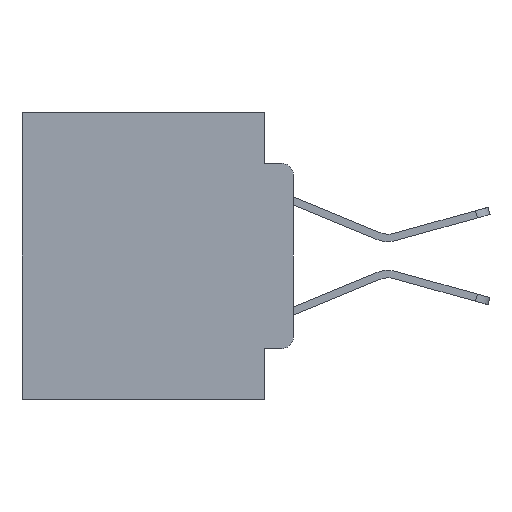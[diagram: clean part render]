
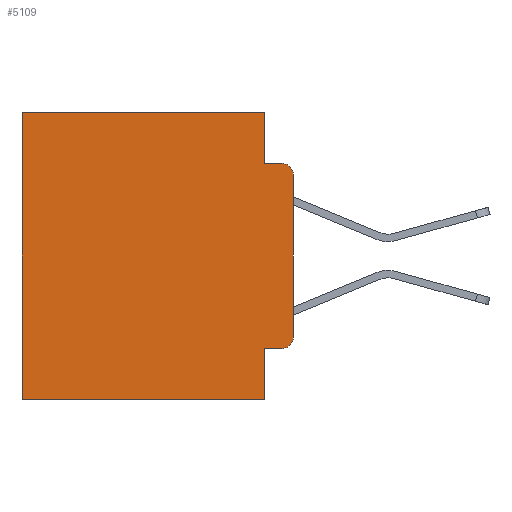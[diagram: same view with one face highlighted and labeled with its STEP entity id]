
A CAD part, left-side view. The second image highlights one B-rep face of the part: STEP entity #5109.
In plain terms, the highlighted planar face has unit normal (-1, 0, 0).
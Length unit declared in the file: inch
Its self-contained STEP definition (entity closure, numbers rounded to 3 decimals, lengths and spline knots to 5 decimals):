
#487 = CARTESIAN_POINT ( 'NONE',  ( 0.298, 0., -0.3915 ) ) ;
#726 = CARTESIAN_POINT ( 'NONE',  ( 0.298, 0.051, -0.4115 ) ) ;
#761 = CARTESIAN_POINT ( 'NONE',  ( 0.298, 0.051, 0. ) ) ;
#1875 = FACE_OUTER_BOUND ( 'NONE', #4667, .T. ) ;
#1947 = CARTESIAN_POINT ( 'NONE',  ( 0.298, 0., 0. ) ) ;
#2018 = PLANE ( 'NONE',  #2571 ) ;
#2416 = VERTEX_POINT ( 'NONE', #8636 ) ;
#2571 = AXIS2_PLACEMENT_3D ( 'NONE', #26349, #21412, #23590 ) ;
#2911 = CARTESIAN_POINT ( 'NONE',  ( 0.298, 0., -0.5 ) ) ;
#3122 = CARTESIAN_POINT ( 'NONE',  ( 0.298, 0.473, 0. ) ) ;
#3281 = DIRECTION ( 'NONE',  ( -1., 0., 0. ) ) ;
#4502 = CARTESIAN_POINT ( 'NONE',  ( 0.298, 0.051, -0.4115 ) ) ;
#4667 = EDGE_LOOP ( 'NONE', ( #11362, #19596, #18901, #5323, #28668, #21080, #15836, #21232, #6042, #21075 ) ) ;
#4672 = EDGE_CURVE ( 'NONE', #19075, #25026, #17510, .T. ) ;
#4812 = VERTEX_POINT ( 'NONE', #4502 ) ;
#4886 = EDGE_CURVE ( 'NONE', #25026, #22188, #6840, .T. ) ;
#4969 = EDGE_CURVE ( 'NONE', #4812, #14832, #7862, .T. ) ;
#5070 = LINE ( 'NONE', #6994, #20782 ) ;
#5094 = CARTESIAN_POINT ( 'NONE',  ( 0.298, 0.02, -0.1085 ) ) ;
#5109 = ADVANCED_FACE ( 'NONE', ( #1875 ), #2018, .F. ) ;
#5323 = ORIENTED_EDGE ( 'NONE', *, *, #4672, .F. ) ;
#5459 = DIRECTION ( 'NONE',  ( 0., 0., -1. ) ) ;
#6042 = ORIENTED_EDGE ( 'NONE', *, *, #4969, .T. ) ;
#6248 = EDGE_CURVE ( 'NONE', #2416, #8622, #24770, .T. ) ;
#6403 = DIRECTION ( 'NONE',  ( 0., 0., -1. ) ) ;
#6766 = CIRCLE ( 'NONE', #7236, 0.02 ) ;
#6840 = LINE ( 'NONE', #15747, #26697 ) ;
#6994 = CARTESIAN_POINT ( 'NONE',  ( 0.298, 0., 0. ) ) ;
#7236 = AXIS2_PLACEMENT_3D ( 'NONE', #17008, #3281, #5459 ) ;
#7862 = LINE ( 'NONE', #726, #8117 ) ;
#8117 = VECTOR ( 'NONE', #18513, 39.37008 ) ;
#8444 = VERTEX_POINT ( 'NONE', #3122 ) ;
#8481 = LINE ( 'NONE', #25953, #27718 ) ;
#8622 = VERTEX_POINT ( 'NONE', #25721 ) ;
#8636 = CARTESIAN_POINT ( 'NONE',  ( 0.298, 0.051, -0.5 ) ) ;
#9099 = VECTOR ( 'NONE', #18489, 39.37008 ) ;
#9623 = LINE ( 'NONE', #11943, #9099 ) ;
#10792 = EDGE_CURVE ( 'NONE', #17193, #22188, #22730, .T. ) ;
#11362 = ORIENTED_EDGE ( 'NONE', *, *, #19406, .F. ) ;
#11943 = CARTESIAN_POINT ( 'NONE',  ( 0.298, 0.473, 0. ) ) ;
#13331 = EDGE_CURVE ( 'NONE', #19075, #8444, #19744, .T. ) ;
#13599 = DIRECTION ( 'NONE',  ( 0., 0., -1. ) ) ;
#14070 = CARTESIAN_POINT ( 'NONE',  ( 0.298, 0.02, -0.4115 ) ) ;
#14832 = VERTEX_POINT ( 'NONE', #14070 ) ;
#15746 = DIRECTION ( 'NONE',  ( 0., 0., -1. ) ) ;
#15747 = CARTESIAN_POINT ( 'NONE',  ( 0.298, 0.051, -0.0885 ) ) ;
#15836 = ORIENTED_EDGE ( 'NONE', *, *, #6248, .F. ) ;
#15892 = EDGE_CURVE ( 'NONE', #8444, #8622, #9623, .T. ) ;
#17008 = CARTESIAN_POINT ( 'NONE',  ( 0.298, 0.02, -0.3915 ) ) ;
#17076 = EDGE_CURVE ( 'NONE', #14832, #20272, #6766, .T. ) ;
#17193 = VERTEX_POINT ( 'NONE', #26169 ) ;
#17510 = LINE ( 'NONE', #28552, #19713 ) ;
#17918 = CARTESIAN_POINT ( 'NONE',  ( 0.298, 0.02, -0.0885 ) ) ;
#18088 = DIRECTION ( 'NONE',  ( 0., 1., 0. ) ) ;
#18489 = DIRECTION ( 'NONE',  ( 0., 0., -1. ) ) ;
#18513 = DIRECTION ( 'NONE',  ( 0., -1., 0. ) ) ;
#18901 = ORIENTED_EDGE ( 'NONE', *, *, #4886, .F. ) ;
#19075 = VERTEX_POINT ( 'NONE', #761 ) ;
#19291 = EDGE_CURVE ( 'NONE', #4812, #2416, #8481, .T. ) ;
#19406 = EDGE_CURVE ( 'NONE', #17193, #20272, #5070, .T. ) ;
#19596 = ORIENTED_EDGE ( 'NONE', *, *, #10792, .T. ) ;
#19701 = DIRECTION ( 'NONE',  ( 0., 0., -1. ) ) ;
#19713 = VECTOR ( 'NONE', #6403, 39.37008 ) ;
#19744 = LINE ( 'NONE', #1947, #26643 ) ;
#20272 = VERTEX_POINT ( 'NONE', #487 ) ;
#20782 = VECTOR ( 'NONE', #15746, 39.37008 ) ;
#21075 = ORIENTED_EDGE ( 'NONE', *, *, #17076, .T. ) ;
#21080 = ORIENTED_EDGE ( 'NONE', *, *, #15892, .T. ) ;
#21232 = ORIENTED_EDGE ( 'NONE', *, *, #19291, .F. ) ;
#21412 = DIRECTION ( 'NONE',  ( 1., 0., 0. ) ) ;
#22188 = VERTEX_POINT ( 'NONE', #17918 ) ;
#22730 = CIRCLE ( 'NONE', #26899, 0.02 ) ;
#23590 = DIRECTION ( 'NONE',  ( 0., 0., -1. ) ) ;
#24612 = DIRECTION ( 'NONE',  ( 0., -1., 0. ) ) ;
#24770 = LINE ( 'NONE', #2911, #26953 ) ;
#24923 = DIRECTION ( 'NONE',  ( -1., 0., 0. ) ) ;
#25026 = VERTEX_POINT ( 'NONE', #28651 ) ;
#25721 = CARTESIAN_POINT ( 'NONE',  ( 0.298, 0.473, -0.5 ) ) ;
#25953 = CARTESIAN_POINT ( 'NONE',  ( 0.298, 0.051, 0. ) ) ;
#26169 = CARTESIAN_POINT ( 'NONE',  ( 0.298, 0., -0.1085 ) ) ;
#26349 = CARTESIAN_POINT ( 'NONE',  ( 0.298, 0., 0. ) ) ;
#26643 = VECTOR ( 'NONE', #28589, 39.37008 ) ;
#26697 = VECTOR ( 'NONE', #24612, 39.37008 ) ;
#26899 = AXIS2_PLACEMENT_3D ( 'NONE', #5094, #24923, #13599 ) ;
#26953 = VECTOR ( 'NONE', #18088, 39.37008 ) ;
#27718 = VECTOR ( 'NONE', #19701, 39.37008 ) ;
#28552 = CARTESIAN_POINT ( 'NONE',  ( 0.298, 0.051, 0. ) ) ;
#28589 = DIRECTION ( 'NONE',  ( 0., 1., 0. ) ) ;
#28651 = CARTESIAN_POINT ( 'NONE',  ( 0.298, 0.051, -0.0885 ) ) ;
#28668 = ORIENTED_EDGE ( 'NONE', *, *, #13331, .T. ) ;
